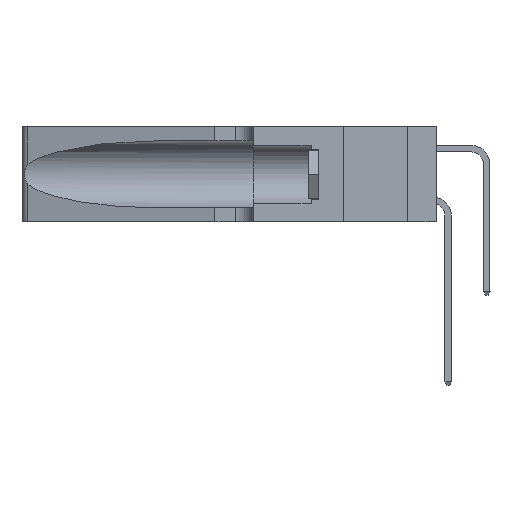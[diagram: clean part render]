
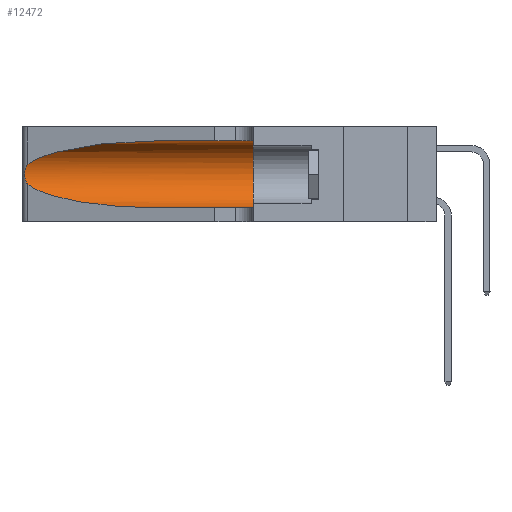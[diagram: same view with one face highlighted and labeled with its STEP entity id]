
A CAD part, left-side view. The second image highlights one B-rep face of the part: STEP entity #12472.
In plain terms, the highlighted cylindrical face has radius 3.308 mm (diameter 6.617 mm), a partial arc.
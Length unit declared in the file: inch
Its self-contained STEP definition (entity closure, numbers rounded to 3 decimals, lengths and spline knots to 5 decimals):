
#526 = DIRECTION ( 'NONE',  ( 0., -1., 0. ) ) ;
#981 = CIRCLE ( 'NONE', #25656, 0.13025 ) ;
#1273 = CARTESIAN_POINT ( 'NONE',  ( 0.25487, 1.22718, 0.14631 ) ) ;
#1362 = CARTESIAN_POINT ( 'NONE',  ( 0.25487, 1.22718, 0.22369 ) ) ;
#1574 = CARTESIAN_POINT ( 'NONE',  ( 0.25789, 1.23486, 0.15765 ) ) ;
#2104 = CARTESIAN_POINT ( 'NONE',  ( 0.1305, 1.61858, 0.05475 ) ) ;
#2770 = CARTESIAN_POINT ( 'NONE',  ( 0.1305, 0.72297, 0.05475 ) ) ;
#3689 =( BOUNDED_CURVE ( )  B_SPLINE_CURVE ( 3, ( #16037, #25782, #25588, #6454 ),
 .UNSPECIFIED., .F., .F. ) 
 B_SPLINE_CURVE_WITH_KNOTS ( ( 4, 4 ),
 ( 1.5708, 2.84003 ),
 .UNSPECIFIED. ) 
 CURVE ( )  GEOMETRIC_REPRESENTATION_ITEM ( )  RATIONAL_B_SPLINE_CURVE ( ( 1., 0.87, 0.87, 1. ) ) 
 REPRESENTATION_ITEM ( '' )  );
#4044 = CARTESIAN_POINT ( 'NONE',  ( 0.25487, 1.22718, 0.14631 ) ) ;
#4362 = DIRECTION ( 'NONE',  ( 0., 0., 1. ) ) ;
#4807 = LINE ( 'NONE', #12612, #21730 ) ;
#5026 = B_SPLINE_CURVE_WITH_KNOTS ( 'NONE', 3,
 ( #1362, #8469, #18059, #25385, #25170, #27994, #13202, #6256, #30088, #16038, #1574, #13516, #25589, #30193 ),
 .UNSPECIFIED., .F., .F.,
 ( 4, 2, 2, 2, 2, 2, 4 ),
 ( 0., 0.00027, 0.00053, 0.00107, 0.0016, 0.00187, 0.00214 ),
 .UNSPECIFIED. ) ;
#5416 = AXIS2_PLACEMENT_3D ( 'NONE', #27076, #526, #12733 ) ;
#6256 = CARTESIAN_POINT ( 'NONE',  ( 0.26075, 1.23896, 0.178 ) ) ;
#6454 = CARTESIAN_POINT ( 'NONE',  ( 0.25487, 1.22718, 0.22369 ) ) ;
#6987 = DIRECTION ( 'NONE',  ( 0., -1., 0. ) ) ;
#8350 = CARTESIAN_POINT ( 'NONE',  ( 0.1305, 0.72297, 0.31525 ) ) ;
#8469 = CARTESIAN_POINT ( 'NONE',  ( 0.25555, 1.22994, 0.2215 ) ) ;
#8527 = ORIENTED_EDGE ( 'NONE', *, *, #16620, .T. ) ;
#9280 = VERTEX_POINT ( 'NONE', #2770 ) ;
#10523 = ORIENTED_EDGE ( 'NONE', *, *, #23182, .F. ) ;
#10683 = CARTESIAN_POINT ( 'NONE',  ( 0.25487, 1.22718, 0.22369 ) ) ;
#10852 = ORIENTED_EDGE ( 'NONE', *, *, #30864, .T. ) ;
#11530 = CARTESIAN_POINT ( 'NONE',  ( 0.1305, 0.72297, 0.05475 ) ) ;
#11825 = DIRECTION ( 'NONE',  ( 0., 1., 0. ) ) ;
#12472 = ADVANCED_FACE ( 'NONE', ( #25871 ), #21381, .F. ) ;
#12506 = DIRECTION ( 'NONE',  ( 0., -1., 0. ) ) ;
#12612 = CARTESIAN_POINT ( 'NONE',  ( 0.1305, 1.61858, 0.31525 ) ) ;
#12733 = DIRECTION ( 'NONE',  ( 0., 0., -1. ) ) ;
#13111 = CARTESIAN_POINT ( 'NONE',  ( 0.1305, 0.35, 0.05475 ) ) ;
#13202 = CARTESIAN_POINT ( 'NONE',  ( 0.26075, 1.23896, 0.19203 ) ) ;
#13516 = CARTESIAN_POINT ( 'NONE',  ( 0.25639, 1.23186, 0.15144 ) ) ;
#13632 = CARTESIAN_POINT ( 'NONE',  ( 0.18966, 0.96281, 0.05475 ) ) ;
#13869 = VECTOR ( 'NONE', #6987, 39.37008 ) ;
#14137 = EDGE_CURVE ( 'NONE', #28561, #24897, #5026, .T. ) ;
#16037 = CARTESIAN_POINT ( 'NONE',  ( 0.1305, 0.72297, 0.31525 ) ) ;
#16038 = CARTESIAN_POINT ( 'NONE',  ( 0.25856, 1.23593, 0.16098 ) ) ;
#16106 = EDGE_LOOP ( 'NONE', ( #27796, #22143, #8527, #10852, #10523, #24230 ) ) ;
#16345 = CARTESIAN_POINT ( 'NONE',  ( 0.2373, 1.15595, 0.08982 ) ) ;
#16454 = VERTEX_POINT ( 'NONE', #16676 ) ;
#16620 = EDGE_CURVE ( 'NONE', #24897, #9280, #26933, .T. ) ;
#16676 = CARTESIAN_POINT ( 'NONE',  ( 0.1305, 0.35, 0.31525 ) ) ;
#17073 = VERTEX_POINT ( 'NONE', #8350 ) ;
#18059 = CARTESIAN_POINT ( 'NONE',  ( 0.25639, 1.23184, 0.21858 ) ) ;
#21381 = CYLINDRICAL_SURFACE ( 'NONE', #5416, 0.13025 ) ;
#21730 = VECTOR ( 'NONE', #12506, 39.37008 ) ;
#22143 = ORIENTED_EDGE ( 'NONE', *, *, #14137, .T. ) ;
#23182 = EDGE_CURVE ( 'NONE', #16454, #24014, #981, .T. ) ;
#23580 = CARTESIAN_POINT ( 'NONE',  ( 0.1305, 0.35, 0.185 ) ) ;
#24014 = VERTEX_POINT ( 'NONE', #13111 ) ;
#24230 = ORIENTED_EDGE ( 'NONE', *, *, #25845, .F. ) ;
#24897 = VERTEX_POINT ( 'NONE', #4044 ) ;
#25170 = CARTESIAN_POINT ( 'NONE',  ( 0.25854, 1.2359, 0.20912 ) ) ;
#25385 = CARTESIAN_POINT ( 'NONE',  ( 0.25787, 1.23484, 0.2124 ) ) ;
#25588 = CARTESIAN_POINT ( 'NONE',  ( 0.2373, 1.15595, 0.28018 ) ) ;
#25589 = CARTESIAN_POINT ( 'NONE',  ( 0.25555, 1.22993, 0.14849 ) ) ;
#25656 = AXIS2_PLACEMENT_3D ( 'NONE', #23580, #11825, #4362 ) ;
#25782 = CARTESIAN_POINT ( 'NONE',  ( 0.18966, 0.96281, 0.31525 ) ) ;
#25845 = EDGE_CURVE ( 'NONE', #17073, #16454, #4807, .T. ) ;
#25871 = FACE_OUTER_BOUND ( 'NONE', #16106, .T. ) ;
#26809 = EDGE_CURVE ( 'NONE', #17073, #28561, #3689, .T. ) ;
#26933 =( BOUNDED_CURVE ( )  B_SPLINE_CURVE ( 3, ( #1273, #16345, #13632, #11530 ),
 .UNSPECIFIED., .F., .T. ) 
 B_SPLINE_CURVE_WITH_KNOTS ( ( 4, 4 ),
 ( 3.44316, 4.71239 ),
 .UNSPECIFIED. ) 
 CURVE ( )  GEOMETRIC_REPRESENTATION_ITEM ( )  RATIONAL_B_SPLINE_CURVE ( ( 1., 0.87, 0.87, 1. ) ) 
 REPRESENTATION_ITEM ( '' )  );
#27076 = CARTESIAN_POINT ( 'NONE',  ( 0.1305, 1.61858, 0.185 ) ) ;
#27371 = LINE ( 'NONE', #2104, #13869 ) ;
#27796 = ORIENTED_EDGE ( 'NONE', *, *, #26809, .T. ) ;
#27994 = CARTESIAN_POINT ( 'NONE',  ( 0.26018, 1.23835, 0.19895 ) ) ;
#28561 = VERTEX_POINT ( 'NONE', #10683 ) ;
#30088 = CARTESIAN_POINT ( 'NONE',  ( 0.26017, 1.23833, 0.17102 ) ) ;
#30193 = CARTESIAN_POINT ( 'NONE',  ( 0.25487, 1.22718, 0.14631 ) ) ;
#30864 = EDGE_CURVE ( 'NONE', #9280, #24014, #27371, .T. ) ;
